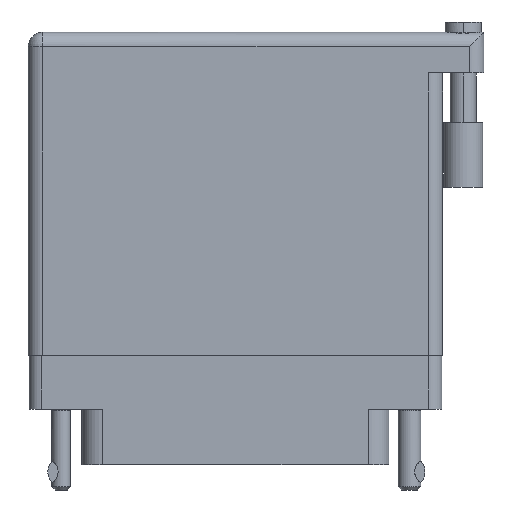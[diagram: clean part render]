
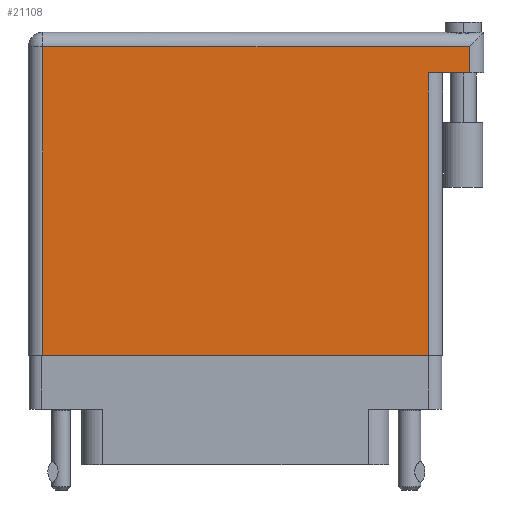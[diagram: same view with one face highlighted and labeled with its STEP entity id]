
A CAD part, front view. The second image highlights one B-rep face of the part: STEP entity #21108.
In plain terms, the highlighted face is planar.
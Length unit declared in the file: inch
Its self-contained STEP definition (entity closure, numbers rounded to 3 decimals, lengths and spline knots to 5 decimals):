
#1474 = CARTESIAN_POINT ( 'NONE',  ( 0., 1.566, 0. ) ) ;
#3251 = LINE ( 'NONE', #32374, #13792 ) ;
#4401 = EDGE_CURVE ( 'NONE', #25962, #20832, #11498, .T. ) ;
#4501 = DIRECTION ( 'NONE',  ( 0., 1., 0. ) ) ;
#4943 = DIRECTION ( 'NONE',  ( -1., 0., 0. ) ) ;
#4965 = EDGE_CURVE ( 'NONE', #43630, #42749, #24169, .T. ) ;
#5005 = VECTOR ( 'NONE', #6833, 39.37008 ) ;
#5408 = LINE ( 'NONE', #41268, #31509 ) ;
#5708 = ORIENTED_EDGE ( 'NONE', *, *, #35152, .T. ) ;
#6833 = DIRECTION ( 'NONE',  ( 1., 0., 0. ) ) ;
#7917 = CARTESIAN_POINT ( 'NONE',  ( 2.138, 1.566, 0. ) ) ;
#8612 = CARTESIAN_POINT ( 'NONE',  ( 2.138, 1.369, 0. ) ) ;
#8927 = DIRECTION ( 'NONE',  ( -1., 0., 0. ) ) ;
#11498 = LINE ( 'NONE', #11951, #36354 ) ;
#11951 = CARTESIAN_POINT ( 'NONE',  ( 2.208, 1.369, 0. ) ) ;
#12735 = DIRECTION ( 'NONE',  ( -1., 0., 0. ) ) ;
#13792 = VECTOR ( 'NONE', #40105, 39.37008 ) ;
#14008 = AXIS2_PLACEMENT_3D ( 'NONE', #1474, #27915, #12735 ) ;
#15255 = CARTESIAN_POINT ( 'NONE',  ( 0.07, 1.496, 0. ) ) ;
#15264 = VERTEX_POINT ( 'NONE', #21025 ) ;
#17163 = VECTOR ( 'NONE', #8927, 39.37008 ) ;
#17474 = EDGE_CURVE ( 'NONE', #25962, #15264, #41027, .T. ) ;
#19546 = ORIENTED_EDGE ( 'NONE', *, *, #20200, .T. ) ;
#20200 = EDGE_CURVE ( 'NONE', #42749, #20832, #3251, .T. ) ;
#20832 = VERTEX_POINT ( 'NONE', #33884 ) ;
#21025 = CARTESIAN_POINT ( 'NONE',  ( 2.138, 1.496, 0. ) ) ;
#21108 = ADVANCED_FACE ( 'NONE', ( #21806 ), #38904, .F. ) ;
#21185 = ORIENTED_EDGE ( 'NONE', *, *, #4965, .T. ) ;
#21806 = FACE_OUTER_BOUND ( 'NONE', #28954, .T. ) ;
#24169 = LINE ( 'NONE', #32771, #5005 ) ;
#25962 = VERTEX_POINT ( 'NONE', #8612 ) ;
#27915 = DIRECTION ( 'NONE',  ( 0., 0., -1. ) ) ;
#28954 = EDGE_LOOP ( 'NONE', ( #21185, #19546, #31194, #46050, #5708, #42020 ) ) ;
#31194 = ORIENTED_EDGE ( 'NONE', *, *, #4401, .F. ) ;
#31229 = VECTOR ( 'NONE', #4501, 39.37008 ) ;
#31509 = VECTOR ( 'NONE', #45161, 39.37008 ) ;
#32374 = CARTESIAN_POINT ( 'NONE',  ( 1.938, 1.369, 0. ) ) ;
#32771 = CARTESIAN_POINT ( 'NONE',  ( 0., 0., 0. ) ) ;
#33884 = CARTESIAN_POINT ( 'NONE',  ( 1.938, 1.369, 0. ) ) ;
#35152 = EDGE_CURVE ( 'NONE', #15264, #38929, #46042, .T. ) ;
#35438 = CARTESIAN_POINT ( 'NONE',  ( 0., 1.496, 0. ) ) ;
#36354 = VECTOR ( 'NONE', #4943, 39.37008 ) ;
#38904 = PLANE ( 'NONE',  #14008 ) ;
#38929 = VERTEX_POINT ( 'NONE', #15255 ) ;
#40105 = DIRECTION ( 'NONE',  ( 0., 1., 0. ) ) ;
#41027 = LINE ( 'NONE', #7917, #31229 ) ;
#41268 = CARTESIAN_POINT ( 'NONE',  ( 0.07, 0., 0. ) ) ;
#42020 = ORIENTED_EDGE ( 'NONE', *, *, #46002, .T. ) ;
#42749 = VERTEX_POINT ( 'NONE', #46415 ) ;
#43630 = VERTEX_POINT ( 'NONE', #46996 ) ;
#45161 = DIRECTION ( 'NONE',  ( 0., -1., 0. ) ) ;
#46002 = EDGE_CURVE ( 'NONE', #38929, #43630, #5408, .T. ) ;
#46042 = LINE ( 'NONE', #35438, #17163 ) ;
#46050 = ORIENTED_EDGE ( 'NONE', *, *, #17474, .T. ) ;
#46415 = CARTESIAN_POINT ( 'NONE',  ( 1.938, 0., 0. ) ) ;
#46996 = CARTESIAN_POINT ( 'NONE',  ( 0.07, 0., 0. ) ) ;
